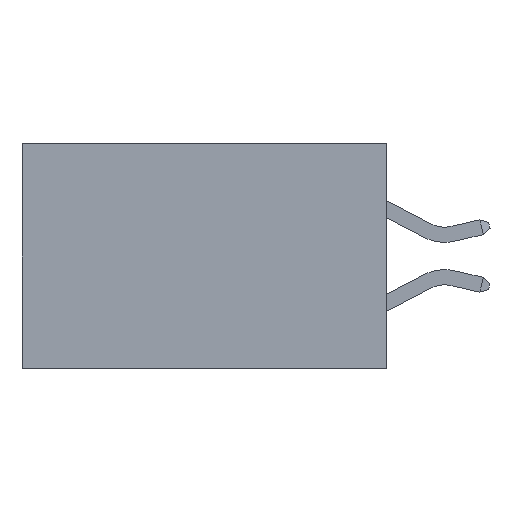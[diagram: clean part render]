
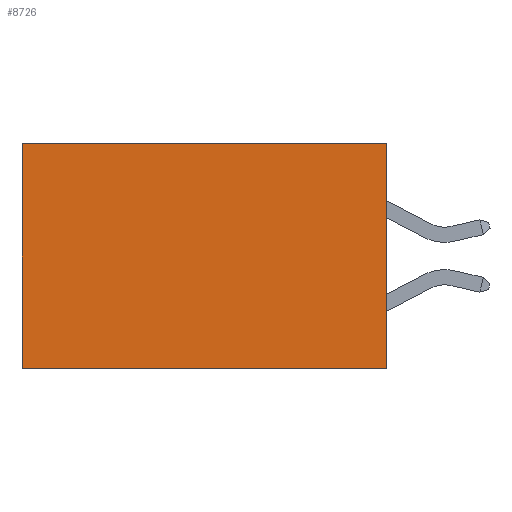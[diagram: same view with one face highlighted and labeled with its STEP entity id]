
A CAD part, left-side view. The second image highlights one B-rep face of the part: STEP entity #8726.
In plain terms, the highlighted planar face has unit normal (-1, 0, 0).
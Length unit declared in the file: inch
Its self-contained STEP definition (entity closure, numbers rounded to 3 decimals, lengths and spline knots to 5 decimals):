
#217 = EDGE_LOOP ( 'NONE', ( #7440, #11300, #16961, #8364 ) ) ;
#893 = LINE ( 'NONE', #2050, #16820 ) ;
#1121 = CARTESIAN_POINT ( 'NONE',  ( 0.2615, 0., 0. ) ) ;
#1157 = AXIS2_PLACEMENT_3D ( 'NONE', #13003, #7591, #17199 ) ;
#1693 = VERTEX_POINT ( 'NONE', #16653 ) ;
#2050 = CARTESIAN_POINT ( 'NONE',  ( 0.2615, 0., -0.37 ) ) ;
#2277 = LINE ( 'NONE', #1121, #5179 ) ;
#3472 = FACE_OUTER_BOUND ( 'NONE', #217, .T. ) ;
#5179 = VECTOR ( 'NONE', #17468, 39.37008 ) ;
#5322 = LINE ( 'NONE', #6383, #7214 ) ;
#5915 = DIRECTION ( 'NONE',  ( 0., 0., -1. ) ) ;
#6383 = CARTESIAN_POINT ( 'NONE',  ( 0.2615, 0.6, -0.37 ) ) ;
#7214 = VECTOR ( 'NONE', #11868, 39.37008 ) ;
#7338 = LINE ( 'NONE', #12938, #16528 ) ;
#7440 = ORIENTED_EDGE ( 'NONE', *, *, #15166, .T. ) ;
#7591 = DIRECTION ( 'NONE',  ( 1., 0., 0. ) ) ;
#8364 = ORIENTED_EDGE ( 'NONE', *, *, #10613, .T. ) ;
#8726 = ADVANCED_FACE ( 'NONE', ( #3472 ), #10189, .F. ) ;
#9540 = VERTEX_POINT ( 'NONE', #14472 ) ;
#10189 = PLANE ( 'NONE',  #1157 ) ;
#10613 = EDGE_CURVE ( 'NONE', #1693, #14689, #2277, .T. ) ;
#11131 = CARTESIAN_POINT ( 'NONE',  ( 0.2615, 0.6, 0. ) ) ;
#11300 = ORIENTED_EDGE ( 'NONE', *, *, #17228, .F. ) ;
#11868 = DIRECTION ( 'NONE',  ( 0., 0., -1. ) ) ;
#12559 = CARTESIAN_POINT ( 'NONE',  ( 0.2615, 0., -0.37 ) ) ;
#12938 = CARTESIAN_POINT ( 'NONE',  ( 0.2615, 0., -0.37 ) ) ;
#13003 = CARTESIAN_POINT ( 'NONE',  ( 0.2615, 0., -0.37 ) ) ;
#13038 = DIRECTION ( 'NONE',  ( 0., 1., 0. ) ) ;
#14472 = CARTESIAN_POINT ( 'NONE',  ( 0.2615, 0.6, -0.37 ) ) ;
#14689 = VERTEX_POINT ( 'NONE', #11131 ) ;
#15166 = EDGE_CURVE ( 'NONE', #14689, #9540, #5322, .T. ) ;
#15431 = EDGE_CURVE ( 'NONE', #1693, #15752, #7338, .T. ) ;
#15752 = VERTEX_POINT ( 'NONE', #12559 ) ;
#16528 = VECTOR ( 'NONE', #5915, 39.37008 ) ;
#16653 = CARTESIAN_POINT ( 'NONE',  ( 0.2615, 0., 0. ) ) ;
#16820 = VECTOR ( 'NONE', #13038, 39.37008 ) ;
#16961 = ORIENTED_EDGE ( 'NONE', *, *, #15431, .F. ) ;
#17199 = DIRECTION ( 'NONE',  ( 0., 0., -1. ) ) ;
#17228 = EDGE_CURVE ( 'NONE', #15752, #9540, #893, .T. ) ;
#17468 = DIRECTION ( 'NONE',  ( 0., 1., 0. ) ) ;
